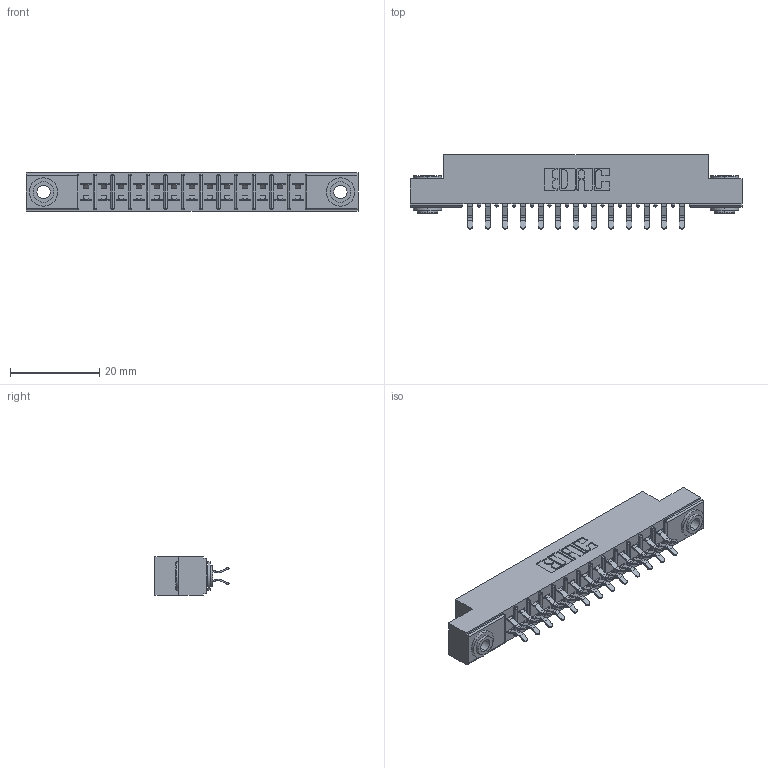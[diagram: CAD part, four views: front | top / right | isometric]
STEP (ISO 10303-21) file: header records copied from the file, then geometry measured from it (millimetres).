
FILE_DESCRIPTION (( 'STEP AP203' ), '1' );
FILE_NAME ('315-026-556-203.STEP', '2019-09-10T15:00:07', ( '' ), ( '' ), 'SwSTEP 2.0', 'SolidWorks 2016', '' );
FILE_SCHEMA (( 'CONFIG_CONTROL_DESIGN' ));
Length unit declared in the file: inch
Products named in the file (4): 315-026-556-203; 305 Part_.156 Dia; 305-290-001_556; 345-250-002_345-250-002-102
Assembly tree (29 placements, depth 2):
  315-026-556-203
    305 Part_.156 Dia
    305-290-001_556  x26
    345-250-002_345-250-002-102  x2
Bounding box: 74.52 x 16.64 x 8.71 mm (x, y, z)
Volume: 4689 mm3; surface area: 8571.1 mm2
Topology: 29 solids, 29 shells, 1624 faces, 4627 edges, 3010 vertices
Faces by surface type: plane 898, cylinder 666, sphere 52, cone 8
Entity records: 18893 total; most frequent: CARTESIAN_POINT 3110, ORIENTED_EDGE 3074, DIRECTION 3051, EDGE_CURVE 1537, LINE 1197, VECTOR 1197, VERTEX_POINT 986, AXIS2_PLACEMENT_3D 927
